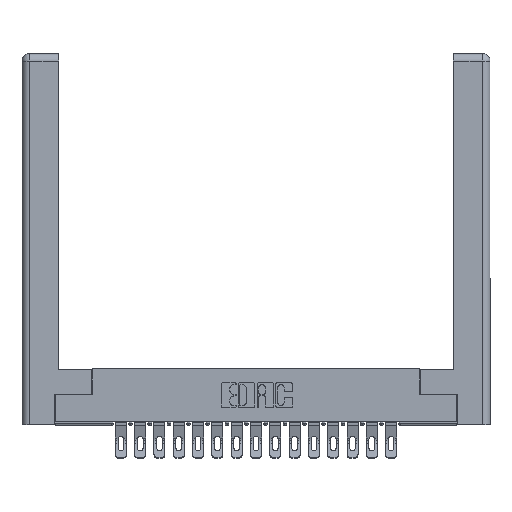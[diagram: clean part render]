
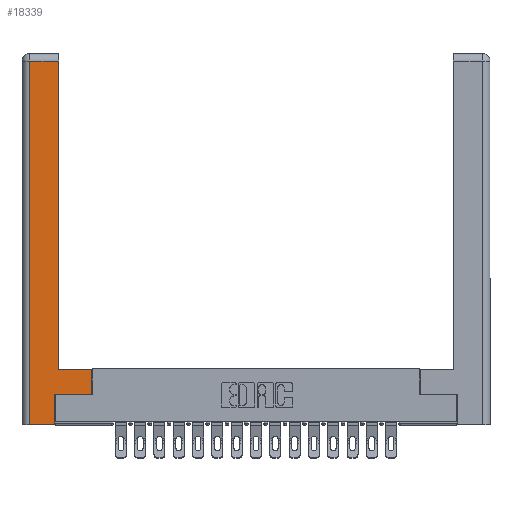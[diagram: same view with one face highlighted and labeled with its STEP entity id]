
A CAD part, top view. The second image highlights one B-rep face of the part: STEP entity #18339.
In plain terms, the highlighted planar face has unit normal (0, 0, 1).
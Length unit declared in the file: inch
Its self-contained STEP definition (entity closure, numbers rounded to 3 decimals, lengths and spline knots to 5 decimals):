
#489 = ORIENTED_EDGE ( 'NONE', *, *, #17191, .T. ) ;
#529 = CARTESIAN_POINT ( 'NONE',  ( 0.265, 0.245, 0. ) ) ;
#741 = VERTEX_POINT ( 'NONE', #11972 ) ;
#896 = VERTEX_POINT ( 'NONE', #21419 ) ;
#1053 = VECTOR ( 'NONE', #21218, 39.37008 ) ;
#1445 = CARTESIAN_POINT ( 'NONE',  ( 0.265, 0., 0. ) ) ;
#2437 = LINE ( 'NONE', #8839, #1053 ) ;
#2615 = DIRECTION ( 'NONE',  ( 1., 0., 0. ) ) ;
#3126 = EDGE_CURVE ( 'NONE', #896, #7167, #6658, .T. ) ;
#3197 = ORIENTED_EDGE ( 'NONE', *, *, #6544, .T. ) ;
#3685 = ORIENTED_EDGE ( 'NONE', *, *, #22794, .T. ) ;
#3890 = DIRECTION ( 'NONE',  ( -1., 0., 0. ) ) ;
#4362 = VERTEX_POINT ( 'NONE', #9744 ) ;
#4422 = CARTESIAN_POINT ( 'NONE',  ( 0.265, 0., 0. ) ) ;
#4986 = DIRECTION ( 'NONE',  ( 0., 0., -1. ) ) ;
#5416 = CARTESIAN_POINT ( 'NONE',  ( 0.295, 0.45, 0. ) ) ;
#5971 = FACE_OUTER_BOUND ( 'NONE', #9052, .T. ) ;
#6272 = LINE ( 'NONE', #15908, #16760 ) ;
#6295 = EDGE_CURVE ( 'NONE', #13763, #4362, #15063, .T. ) ;
#6507 = ORIENTED_EDGE ( 'NONE', *, *, #6295, .T. ) ;
#6538 = VECTOR ( 'NONE', #21708, 39.37008 ) ;
#6544 = EDGE_CURVE ( 'NONE', #741, #896, #7928, .T. ) ;
#6658 = LINE ( 'NONE', #21592, #16309 ) ;
#6877 = VECTOR ( 'NONE', #2615, 39.37008 ) ;
#6894 = CARTESIAN_POINT ( 'NONE',  ( 0., 0., 0. ) ) ;
#7146 = ORIENTED_EDGE ( 'NONE', *, *, #3126, .T. ) ;
#7167 = VERTEX_POINT ( 'NONE', #17650 ) ;
#7428 = VECTOR ( 'NONE', #3890, 39.37008 ) ;
#7928 = LINE ( 'NONE', #15405, #13149 ) ;
#8839 = CARTESIAN_POINT ( 'NONE',  ( 0.565, 0.45, 0. ) ) ;
#9052 = EDGE_LOOP ( 'NONE', ( #15029, #3197, #7146, #3685, #6507, #16408, #13108, #489 ) ) ;
#9162 = CARTESIAN_POINT ( 'NONE',  ( 0.565, 0.45, 0. ) ) ;
#9414 = VECTOR ( 'NONE', #22393, 39.37008 ) ;
#9744 = CARTESIAN_POINT ( 'NONE',  ( 0.265, 0.245, 0. ) ) ;
#10931 = VERTEX_POINT ( 'NONE', #9162 ) ;
#10973 = LINE ( 'NONE', #5416, #7428 ) ;
#10986 = DIRECTION ( 'NONE',  ( 0., -1., 0. ) ) ;
#11845 = DIRECTION ( 'NONE',  ( -1., 0., 0. ) ) ;
#11972 = CARTESIAN_POINT ( 'NONE',  ( 0.295, 2.94, 0. ) ) ;
#13058 = EDGE_CURVE ( 'NONE', #15850, #741, #17996, .T. ) ;
#13108 = ORIENTED_EDGE ( 'NONE', *, *, #18731, .T. ) ;
#13149 = VECTOR ( 'NONE', #11845, 39.37008 ) ;
#13763 = VERTEX_POINT ( 'NONE', #1445 ) ;
#14799 = VERTEX_POINT ( 'NONE', #17569 ) ;
#15029 = ORIENTED_EDGE ( 'NONE', *, *, #13058, .T. ) ;
#15063 = LINE ( 'NONE', #529, #6538 ) ;
#15304 = CARTESIAN_POINT ( 'NONE',  ( 0.295, 0.45, 0. ) ) ;
#15405 = CARTESIAN_POINT ( 'NONE',  ( 0.0615, 2.94, 0. ) ) ;
#15470 = EDGE_CURVE ( 'NONE', #4362, #14799, #6272, .T. ) ;
#15668 = PLANE ( 'NONE',  #16068 ) ;
#15749 = DIRECTION ( 'NONE',  ( -1., 0., 0. ) ) ;
#15850 = VERTEX_POINT ( 'NONE', #15304 ) ;
#15908 = CARTESIAN_POINT ( 'NONE',  ( 0.565, 0.245, 0. ) ) ;
#16068 = AXIS2_PLACEMENT_3D ( 'NONE', #6894, #4986, #15749 ) ;
#16309 = VECTOR ( 'NONE', #10986, 39.37008 ) ;
#16408 = ORIENTED_EDGE ( 'NONE', *, *, #15470, .T. ) ;
#16760 = VECTOR ( 'NONE', #18251, 39.37008 ) ;
#17191 = EDGE_CURVE ( 'NONE', #10931, #15850, #10973, .T. ) ;
#17358 = LINE ( 'NONE', #4422, #6877 ) ;
#17569 = CARTESIAN_POINT ( 'NONE',  ( 0.565, 0.245, 0. ) ) ;
#17650 = CARTESIAN_POINT ( 'NONE',  ( 0.0615, 0., 0. ) ) ;
#17996 = LINE ( 'NONE', #22022, #9414 ) ;
#18251 = DIRECTION ( 'NONE',  ( 1., 0., 0. ) ) ;
#18339 = ADVANCED_FACE ( 'NONE', ( #5971 ), #15668, .F. ) ;
#18731 = EDGE_CURVE ( 'NONE', #14799, #10931, #2437, .T. ) ;
#21218 = DIRECTION ( 'NONE',  ( 0., 1., 0. ) ) ;
#21419 = CARTESIAN_POINT ( 'NONE',  ( 0.0615, 2.94, 0. ) ) ;
#21592 = CARTESIAN_POINT ( 'NONE',  ( 0.0615, 0., 0. ) ) ;
#21708 = DIRECTION ( 'NONE',  ( 0., 1., 0. ) ) ;
#22022 = CARTESIAN_POINT ( 'NONE',  ( 0.295, 3., 0. ) ) ;
#22393 = DIRECTION ( 'NONE',  ( 0., 1., 0. ) ) ;
#22794 = EDGE_CURVE ( 'NONE', #7167, #13763, #17358, .T. ) ;
